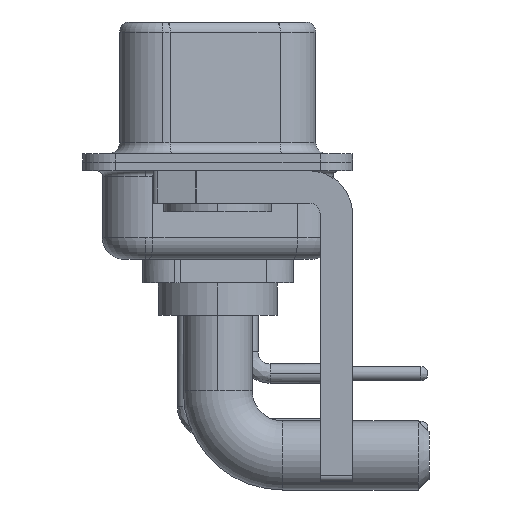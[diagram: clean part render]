
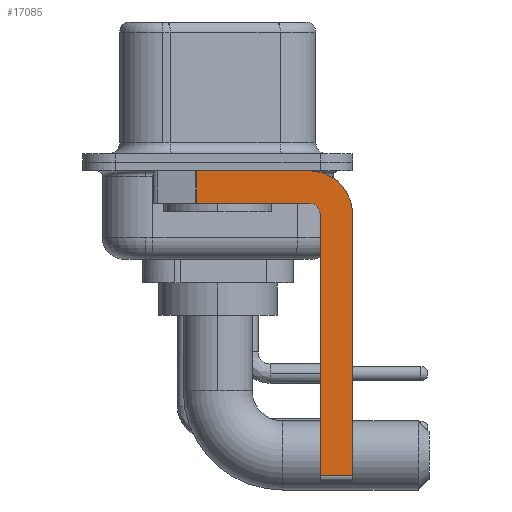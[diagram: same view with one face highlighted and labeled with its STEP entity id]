
A CAD part, left-side view. The second image highlights one B-rep face of the part: STEP entity #17085.
In plain terms, the highlighted planar face has unit normal (-1, 0, 0).
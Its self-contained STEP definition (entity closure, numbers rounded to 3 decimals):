
#1381 = ORIENTED_EDGE ( 'NONE', *, *, #2896, .F. ) ;
#1433 = VECTOR ( 'NONE', #8895, 1000. ) ;
#1474 = LINE ( 'NONE', #9257, #21346 ) ;
#1631 = CARTESIAN_POINT ( 'NONE',  ( -2.9, -4.75, -14.55 ) ) ;
#1681 = VECTOR ( 'NONE', #18508, 1000. ) ;
#1916 = CARTESIAN_POINT ( 'NONE',  ( -2.9, -6.25, -2.4 ) ) ;
#2118 = AXIS2_PLACEMENT_3D ( 'NONE', #14046, #21582, #8302 ) ;
#2697 = LINE ( 'NONE', #6773, #1681 ) ;
#2896 = EDGE_CURVE ( 'NONE', #21568, #22935, #9866, .T. ) ;
#3152 = LINE ( 'NONE', #16302, #1433 ) ;
#3312 = VERTEX_POINT ( 'NONE', #16899 ) ;
#3746 = AXIS2_PLACEMENT_3D ( 'NONE', #16983, #20957, #9326 ) ;
#3943 = DIRECTION ( 'NONE',  ( 0., 0., -1. ) ) ;
#4513 = DIRECTION ( 'NONE',  ( 0., 0., 1. ) ) ;
#4936 = EDGE_CURVE ( 'NONE', #23242, #5506, #9217, .T. ) ;
#5506 = VERTEX_POINT ( 'NONE', #17288 ) ;
#5596 = DIRECTION ( 'NONE',  ( 1., 0., 0. ) ) ;
#6269 = CIRCLE ( 'NONE', #20534, 2. ) ;
#6773 = CARTESIAN_POINT ( 'NONE',  ( -2.9, -4.25, -1.9 ) ) ;
#7556 = DIRECTION ( 'NONE',  ( 0., 0., -1. ) ) ;
#8175 = EDGE_CURVE ( 'NONE', #23242, #3312, #12186, .T. ) ;
#8302 = DIRECTION ( 'NONE',  ( 0., 0., -1. ) ) ;
#8379 = VERTEX_POINT ( 'NONE', #13447 ) ;
#8528 = ORIENTED_EDGE ( 'NONE', *, *, #22077, .F. ) ;
#8895 = DIRECTION ( 'NONE',  ( 0., -1., 0. ) ) ;
#9134 = EDGE_CURVE ( 'NONE', #22935, #5506, #2697, .T. ) ;
#9217 = LINE ( 'NONE', #21091, #11946 ) ;
#9257 = CARTESIAN_POINT ( 'NONE',  ( -2.9, -6.25, -2.4 ) ) ;
#9294 = CARTESIAN_POINT ( 'NONE',  ( -2.9, -4.25, -2.4 ) ) ;
#9326 = DIRECTION ( 'NONE',  ( 0., 0., 1. ) ) ;
#9866 = CIRCLE ( 'NONE', #3746, 0.5 ) ;
#10291 = CARTESIAN_POINT ( 'NONE',  ( -2.9, 3., -0.4 ) ) ;
#11303 = EDGE_CURVE ( 'NONE', #3312, #15833, #6269, .T. ) ;
#11339 = EDGE_LOOP ( 'NONE', ( #15633, #12334, #16446, #1381, #8528, #19051, #11761, #21161 ) ) ;
#11761 = ORIENTED_EDGE ( 'NONE', *, *, #14771, .F. ) ;
#11946 = VECTOR ( 'NONE', #7556, 1000. ) ;
#12186 = LINE ( 'NONE', #10291, #23119 ) ;
#12227 = CARTESIAN_POINT ( 'NONE',  ( -2.9, 0.978, -0.4 ) ) ;
#12334 = ORIENTED_EDGE ( 'NONE', *, *, #4936, .T. ) ;
#13447 = CARTESIAN_POINT ( 'NONE',  ( -2.9, -6.25, -14.55 ) ) ;
#14046 = CARTESIAN_POINT ( 'NONE',  ( -2.9, -4.25, -2.4 ) ) ;
#14083 = LINE ( 'NONE', #18035, #19902 ) ;
#14771 = EDGE_CURVE ( 'NONE', #15833, #8379, #1474, .T. ) ;
#15633 = ORIENTED_EDGE ( 'NONE', *, *, #8175, .F. ) ;
#15833 = VERTEX_POINT ( 'NONE', #1916 ) ;
#16302 = CARTESIAN_POINT ( 'NONE',  ( -2.9, -4.25, -14.55 ) ) ;
#16446 = ORIENTED_EDGE ( 'NONE', *, *, #9134, .F. ) ;
#16899 = CARTESIAN_POINT ( 'NONE',  ( -2.9, -4.25, -0.4 ) ) ;
#16983 = CARTESIAN_POINT ( 'NONE',  ( -2.9, -4.25, -2.4 ) ) ;
#17085 = ADVANCED_FACE ( 'NONE', ( #21843 ), #17489, .F. ) ;
#17288 = CARTESIAN_POINT ( 'NONE',  ( -2.9, 0.978, -1.9 ) ) ;
#17489 = PLANE ( 'NONE',  #2118 ) ;
#17935 = DIRECTION ( 'NONE',  ( 0., -1., 0. ) ) ;
#18035 = CARTESIAN_POINT ( 'NONE',  ( -2.9, -4.75, -14.8 ) ) ;
#18508 = DIRECTION ( 'NONE',  ( 0., 1., 0. ) ) ;
#19051 = ORIENTED_EDGE ( 'NONE', *, *, #19869, .T. ) ;
#19869 = EDGE_CURVE ( 'NONE', #23522, #8379, #3152, .T. ) ;
#19902 = VECTOR ( 'NONE', #4513, 1000. ) ;
#20127 = CARTESIAN_POINT ( 'NONE',  ( -2.9, -4.75, -2.4 ) ) ;
#20534 = AXIS2_PLACEMENT_3D ( 'NONE', #9294, #5596, #3943 ) ;
#20567 = CARTESIAN_POINT ( 'NONE',  ( -2.9, -4.25, -1.9 ) ) ;
#20957 = DIRECTION ( 'NONE',  ( -1., 0., 0. ) ) ;
#21091 = CARTESIAN_POINT ( 'NONE',  ( -2.9, 0.978, -1.9 ) ) ;
#21161 = ORIENTED_EDGE ( 'NONE', *, *, #11303, .F. ) ;
#21346 = VECTOR ( 'NONE', #24840, 1000. ) ;
#21568 = VERTEX_POINT ( 'NONE', #20127 ) ;
#21582 = DIRECTION ( 'NONE',  ( 1., 0., 0. ) ) ;
#21843 = FACE_OUTER_BOUND ( 'NONE', #11339, .T. ) ;
#22077 = EDGE_CURVE ( 'NONE', #23522, #21568, #14083, .T. ) ;
#22935 = VERTEX_POINT ( 'NONE', #20567 ) ;
#23119 = VECTOR ( 'NONE', #17935, 1000. ) ;
#23242 = VERTEX_POINT ( 'NONE', #12227 ) ;
#23522 = VERTEX_POINT ( 'NONE', #1631 ) ;
#24840 = DIRECTION ( 'NONE',  ( 0., 0., -1. ) ) ;
